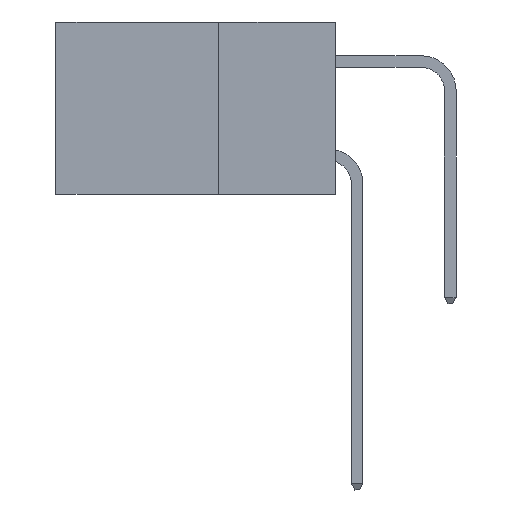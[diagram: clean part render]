
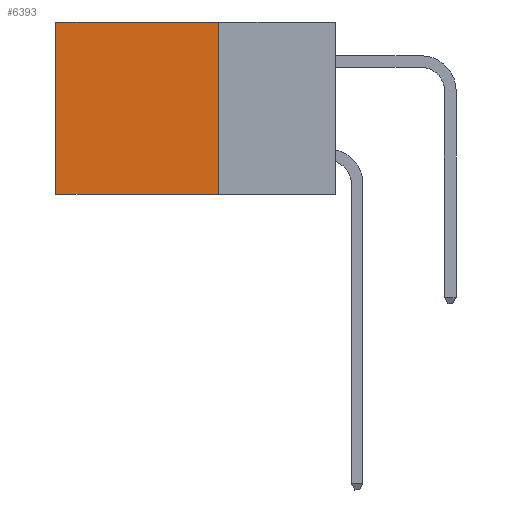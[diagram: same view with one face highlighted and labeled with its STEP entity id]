
A CAD part, left-side view. The second image highlights one B-rep face of the part: STEP entity #6393.
In plain terms, the highlighted planar face has unit normal (-1, 0, 0).
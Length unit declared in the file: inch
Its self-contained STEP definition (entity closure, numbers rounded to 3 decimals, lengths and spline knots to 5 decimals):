
#19 = EDGE_LOOP ( 'NONE', ( #6479, #1252, #6051, #2666 ) ) ;
#474 = VERTEX_POINT ( 'NONE', #6049 ) ;
#609 = CARTESIAN_POINT ( 'NONE',  ( 0.2875, 0.6, 0. ) ) ;
#866 = CARTESIAN_POINT ( 'NONE',  ( 0.2875, 0.6, -0.37 ) ) ;
#992 = EDGE_CURVE ( 'NONE', #474, #8724, #1001, .T. ) ;
#1001 = LINE ( 'NONE', #1566, #3720 ) ;
#1162 = CARTESIAN_POINT ( 'NONE',  ( 0.2875, 0.6, 0. ) ) ;
#1252 = ORIENTED_EDGE ( 'NONE', *, *, #1509, .F. ) ;
#1509 = EDGE_CURVE ( 'NONE', #2087, #4368, #9433, .T. ) ;
#1566 = CARTESIAN_POINT ( 'NONE',  ( 0.2875, 0.25, 0. ) ) ;
#2087 = VERTEX_POINT ( 'NONE', #9170 ) ;
#2280 = DIRECTION ( 'NONE',  ( 0., 0., -1. ) ) ;
#2666 = ORIENTED_EDGE ( 'NONE', *, *, #992, .T. ) ;
#3151 = DIRECTION ( 'NONE',  ( 0., 0., -1. ) ) ;
#3720 = VECTOR ( 'NONE', #4513, 39.37008 ) ;
#4007 = DIRECTION ( 'NONE',  ( 1., 0., 0. ) ) ;
#4368 = VERTEX_POINT ( 'NONE', #866 ) ;
#4513 = DIRECTION ( 'NONE',  ( 0., 1., 0. ) ) ;
#4618 = AXIS2_PLACEMENT_3D ( 'NONE', #9491, #4007, #2280 ) ;
#6049 = CARTESIAN_POINT ( 'NONE',  ( 0.2875, 0.25, 0. ) ) ;
#6051 = ORIENTED_EDGE ( 'NONE', *, *, #10918, .F. ) ;
#6393 = ADVANCED_FACE ( 'NONE', ( #6907 ), #10482, .F. ) ;
#6479 = ORIENTED_EDGE ( 'NONE', *, *, #10691, .T. ) ;
#6907 = FACE_OUTER_BOUND ( 'NONE', #19, .T. ) ;
#7378 = DIRECTION ( 'NONE',  ( 0., 1., 0. ) ) ;
#7440 = DIRECTION ( 'NONE',  ( 0., 0., -1. ) ) ;
#8373 = CARTESIAN_POINT ( 'NONE',  ( 0.2875, 0.25, -0.37 ) ) ;
#8724 = VERTEX_POINT ( 'NONE', #609 ) ;
#9170 = CARTESIAN_POINT ( 'NONE',  ( 0.2875, 0.25, -0.37 ) ) ;
#9389 = LINE ( 'NONE', #11352, #10668 ) ;
#9433 = LINE ( 'NONE', #8373, #9705 ) ;
#9491 = CARTESIAN_POINT ( 'NONE',  ( 0.2875, 0.25, 0. ) ) ;
#9705 = VECTOR ( 'NONE', #7378, 39.37008 ) ;
#10482 = PLANE ( 'NONE',  #4618 ) ;
#10668 = VECTOR ( 'NONE', #3151, 39.37008 ) ;
#10691 = EDGE_CURVE ( 'NONE', #8724, #4368, #11537, .T. ) ;
#10918 = EDGE_CURVE ( 'NONE', #474, #2087, #9389, .T. ) ;
#11352 = CARTESIAN_POINT ( 'NONE',  ( 0.2875, 0.25, 0. ) ) ;
#11372 = VECTOR ( 'NONE', #7440, 39.37008 ) ;
#11537 = LINE ( 'NONE', #1162, #11372 ) ;
